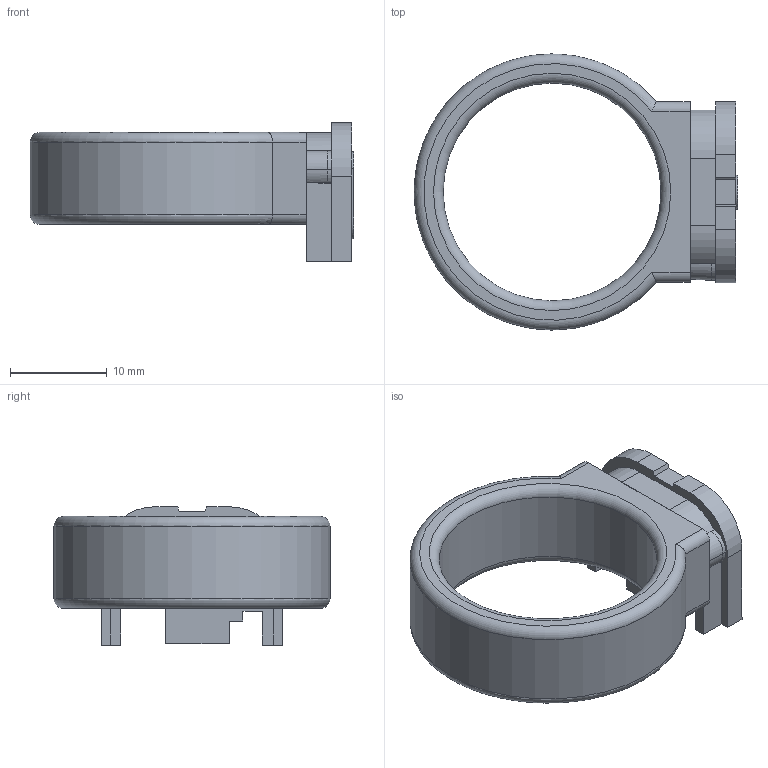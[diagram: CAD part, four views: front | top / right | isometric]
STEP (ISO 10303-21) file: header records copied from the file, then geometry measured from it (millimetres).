
FILE_DESCRIPTION(/* description */ (''),/* implementation_level */ '2;1');
FILE_NAME(/* name */ 'Glocknofsky Charging Ring (No Hardware) v1 final.step',/* time_stamp */ '2022-04-10T11:50:51-04:00',/* author */ (''),/* organization */ (''),/* preprocessor_version */ 'ST-DEVELOPER v18.1',/* originating_system */ 'Autodesk Translation Framework v10.14.0.1471',/* authorisation */ '');
FILE_SCHEMA (('AUTOMOTIVE_DESIGN { 1 0 10303 214 3 1 1 }'));
Length unit declared in the file: millimetre
Products named in the file (1): Glocknofsky Charging Ring (No Hardware)
Bounding box: 33.43 x 28.5 x 14.3 mm (x, y, z)
Volume: 3355.9 mm3; surface area: 2477.6 mm2
Topology: 1 solids, 1 shells, 57 faces, 154 edges, 100 vertices
Faces by surface type: plane 36, cylinder 15, torus 4, bspline 2
Full cylindrical faces by diameter (mm): 22.5 x1
Entity records: 1876 total; most frequent: CARTESIAN_POINT 380, ORIENTED_EDGE 308, DIRECTION 299, EDGE_CURVE 154, LINE 111, VECTOR 111, VERTEX_POINT 100, AXIS2_PLACEMENT_3D 94
